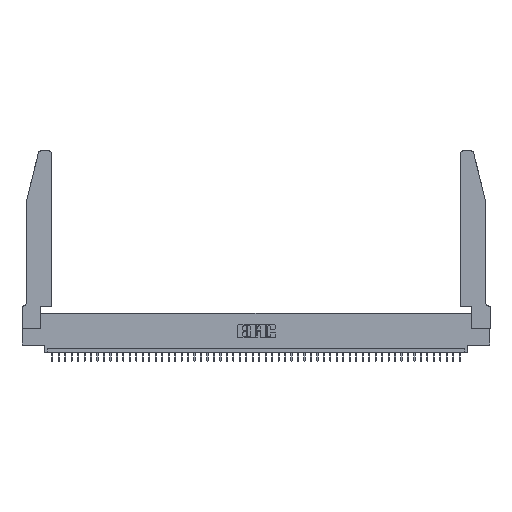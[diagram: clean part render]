
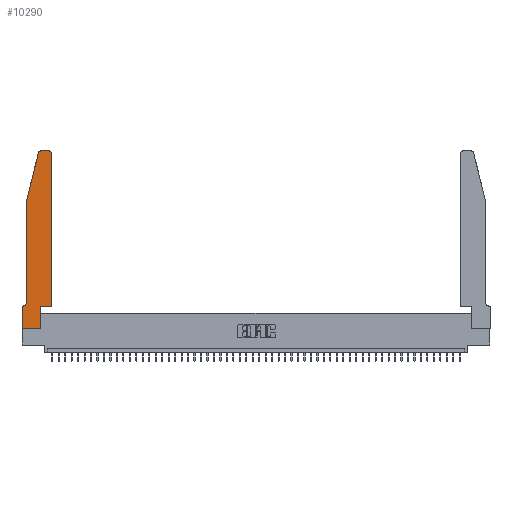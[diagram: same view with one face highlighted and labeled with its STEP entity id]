
A CAD part, top view. The second image highlights one B-rep face of the part: STEP entity #10290.
In plain terms, the highlighted planar face has unit normal (0, 0, 1).
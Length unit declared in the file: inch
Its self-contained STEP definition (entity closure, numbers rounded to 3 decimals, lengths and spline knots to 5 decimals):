
#46 = VECTOR ( 'NONE', #41802, 39.37008 ) ;
#1073 = VECTOR ( 'NONE', #48157, 39.37008 ) ;
#1938 = CARTESIAN_POINT ( 'NONE',  ( 0.2865, 0.35, 0.37 ) ) ;
#2012 = CARTESIAN_POINT ( 'NONE',  ( 0., 0.35, 0.37 ) ) ;
#2520 = VERTEX_POINT ( 'NONE', #20907 ) ;
#2843 = VERTEX_POINT ( 'NONE', #37907 ) ;
#3759 = EDGE_CURVE ( 'NONE', #44016, #2843, #11005, .T. ) ;
#5109 = VECTOR ( 'NONE', #26558, 39.37008 ) ;
#6058 = FACE_OUTER_BOUND ( 'NONE', #34387, .T. ) ;
#6128 = EDGE_CURVE ( 'NONE', #6857, #20717, #10007, .T. ) ;
#6669 = VERTEX_POINT ( 'NONE', #6891 ) ;
#6696 = AXIS2_PLACEMENT_3D ( 'NONE', #35033, #38353, #7597 ) ;
#6857 = VERTEX_POINT ( 'NONE', #25668 ) ;
#6891 = CARTESIAN_POINT ( 'NONE',  ( 0.25487, 2.72718, 0.37 ) ) ;
#6933 = CARTESIAN_POINT ( 'NONE',  ( 0.0755, 2., 0.37 ) ) ;
#7264 = DIRECTION ( 'NONE',  ( 0., 1., 0. ) ) ;
#7509 = ORIENTED_EDGE ( 'NONE', *, *, #19152, .T. ) ;
#7597 = DIRECTION ( 'NONE',  ( 1., 0., 0. ) ) ;
#8338 = ORIENTED_EDGE ( 'NONE', *, *, #40471, .T. ) ;
#8549 = VECTOR ( 'NONE', #49089, 39.37008 ) ;
#8904 = AXIS2_PLACEMENT_3D ( 'NONE', #31086, #23251, #12030 ) ;
#9555 = CARTESIAN_POINT ( 'NONE',  ( 0.4505, 0.35, 0.37 ) ) ;
#10007 = LINE ( 'NONE', #14087, #23589 ) ;
#10290 = ADVANCED_FACE ( 'NONE', ( #6058 ), #36822, .T. ) ;
#11005 = LINE ( 'NONE', #6933, #32248 ) ;
#12030 = DIRECTION ( 'NONE',  ( 1., 0., 0. ) ) ;
#12547 = CARTESIAN_POINT ( 'NONE',  ( 0.2865, 0., 0.37 ) ) ;
#13340 = EDGE_CURVE ( 'NONE', #2520, #31017, #27591, .T. ) ;
#14087 = CARTESIAN_POINT ( 'NONE',  ( 0., 0., 0.37 ) ) ;
#16079 = DIRECTION ( 'NONE',  ( -1., 0., 0. ) ) ;
#16494 = ORIENTED_EDGE ( 'NONE', *, *, #3759, .T. ) ;
#16759 = DIRECTION ( 'NONE',  ( 1., 0., 0. ) ) ;
#17531 = CIRCLE ( 'NONE', #49150, 0.07 ) ;
#17590 = CARTESIAN_POINT ( 'NONE',  ( 0.4505, 0.35, 0.37 ) ) ;
#18054 = VECTOR ( 'NONE', #33067, 39.37008 ) ;
#18724 = CARTESIAN_POINT ( 'NONE',  ( 0.0055, 0.42, 0.37 ) ) ;
#19033 = ORIENTED_EDGE ( 'NONE', *, *, #35173, .T. ) ;
#19152 = EDGE_CURVE ( 'NONE', #48917, #32915, #34416, .T. ) ;
#19551 = ORIENTED_EDGE ( 'NONE', *, *, #39757, .T. ) ;
#19602 = VECTOR ( 'NONE', #16079, 39.37008 ) ;
#19843 = CARTESIAN_POINT ( 'NONE',  ( 0.0055, 0.35, 0.37 ) ) ;
#20717 = VERTEX_POINT ( 'NONE', #12547 ) ;
#20907 = CARTESIAN_POINT ( 'NONE',  ( 0.4505, 2.72, 0.37 ) ) ;
#23020 = LINE ( 'NONE', #34917, #46 ) ;
#23251 = DIRECTION ( 'NONE',  ( 0., 0., 1. ) ) ;
#23589 = VECTOR ( 'NONE', #49363, 39.37008 ) ;
#24156 = VERTEX_POINT ( 'NONE', #39076 ) ;
#25668 = CARTESIAN_POINT ( 'NONE',  ( 0., 0., 0.37 ) ) ;
#26558 = DIRECTION ( 'NONE',  ( -1., 0., 0. ) ) ;
#27591 = CIRCLE ( 'NONE', #8904, 0.03 ) ;
#28416 = EDGE_CURVE ( 'NONE', #6669, #44016, #32864, .T. ) ;
#28615 = CIRCLE ( 'NONE', #6696, 0.03 ) ;
#31017 = VERTEX_POINT ( 'NONE', #31880 ) ;
#31086 = CARTESIAN_POINT ( 'NONE',  ( 0.4205, 2.72, 0.37 ) ) ;
#31209 = ORIENTED_EDGE ( 'NONE', *, *, #13340, .T. ) ;
#31309 = ORIENTED_EDGE ( 'NONE', *, *, #28416, .T. ) ;
#31570 = CARTESIAN_POINT ( 'NONE',  ( 0.2605, 2.75, 0.37 ) ) ;
#31880 = CARTESIAN_POINT ( 'NONE',  ( 0.4205, 2.75, 0.37 ) ) ;
#32248 = VECTOR ( 'NONE', #49350, 39.37008 ) ;
#32677 = LINE ( 'NONE', #44604, #1073 ) ;
#32864 = LINE ( 'NONE', #36936, #8549 ) ;
#32915 = VERTEX_POINT ( 'NONE', #45229 ) ;
#33067 = DIRECTION ( 'NONE',  ( 1., 0., 0. ) ) ;
#34271 = CARTESIAN_POINT ( 'NONE',  ( 0.0755, 2., 0.37 ) ) ;
#34387 = EDGE_LOOP ( 'NONE', ( #38650, #19551, #31309, #16494, #44761, #7509, #19033, #42016, #8338, #45963, #37412, #31209 ) ) ;
#34416 = LINE ( 'NONE', #37974, #5109 ) ;
#34711 = LINE ( 'NONE', #49193, #45926 ) ;
#34917 = CARTESIAN_POINT ( 'NONE',  ( 0., 0., 0.37 ) ) ;
#35033 = CARTESIAN_POINT ( 'NONE',  ( 0.284, 2.72, 0.37 ) ) ;
#35173 = EDGE_CURVE ( 'NONE', #32915, #6857, #23020, .T. ) ;
#36822 = PLANE ( 'NONE',  #45230 ) ;
#36936 = CARTESIAN_POINT ( 'NONE',  ( 0.0755, 2., 0.37 ) ) ;
#37412 = ORIENTED_EDGE ( 'NONE', *, *, #45653, .T. ) ;
#37907 = CARTESIAN_POINT ( 'NONE',  ( 0.0755, 0.42, 0.37 ) ) ;
#37974 = CARTESIAN_POINT ( 'NONE',  ( 0.0755, 0.35, 0.37 ) ) ;
#38353 = DIRECTION ( 'NONE',  ( 0., 0., 1. ) ) ;
#38650 = ORIENTED_EDGE ( 'NONE', *, *, #48600, .T. ) ;
#38900 = EDGE_CURVE ( 'NONE', #40502, #40506, #40430, .T. ) ;
#39076 = CARTESIAN_POINT ( 'NONE',  ( 0.284, 2.75, 0.37 ) ) ;
#39757 = EDGE_CURVE ( 'NONE', #24156, #6669, #28615, .T. ) ;
#40430 = LINE ( 'NONE', #17590, #18054 ) ;
#40471 = EDGE_CURVE ( 'NONE', #20717, #40502, #32677, .T. ) ;
#40502 = VERTEX_POINT ( 'NONE', #1938 ) ;
#40506 = VERTEX_POINT ( 'NONE', #9555 ) ;
#41802 = DIRECTION ( 'NONE',  ( 0., -1., 0. ) ) ;
#42016 = ORIENTED_EDGE ( 'NONE', *, *, #6128, .T. ) ;
#43129 = EDGE_CURVE ( 'NONE', #2843, #48917, #17531, .T. ) ;
#43909 = DIRECTION ( 'NONE',  ( 0., 0., 1. ) ) ;
#44016 = VERTEX_POINT ( 'NONE', #34271 ) ;
#44604 = CARTESIAN_POINT ( 'NONE',  ( 0.2865, 0.35, 0.37 ) ) ;
#44761 = ORIENTED_EDGE ( 'NONE', *, *, #43129, .T. ) ;
#45229 = CARTESIAN_POINT ( 'NONE',  ( 0., 0.35, 0.37 ) ) ;
#45230 = AXIS2_PLACEMENT_3D ( 'NONE', #2012, #43909, #16759 ) ;
#45653 = EDGE_CURVE ( 'NONE', #40506, #2520, #34711, .T. ) ;
#45926 = VECTOR ( 'NONE', #7264, 39.37008 ) ;
#45963 = ORIENTED_EDGE ( 'NONE', *, *, #38900, .T. ) ;
#46108 = DIRECTION ( 'NONE',  ( -1., 0., 0. ) ) ;
#46358 = DIRECTION ( 'NONE',  ( 0., 0., -1. ) ) ;
#46554 = LINE ( 'NONE', #31570, #19602 ) ;
#48157 = DIRECTION ( 'NONE',  ( 0., 1., 0. ) ) ;
#48600 = EDGE_CURVE ( 'NONE', #31017, #24156, #46554, .T. ) ;
#48917 = VERTEX_POINT ( 'NONE', #19843 ) ;
#49089 = DIRECTION ( 'NONE',  ( -0.239, -0.971, 0. ) ) ;
#49150 = AXIS2_PLACEMENT_3D ( 'NONE', #18724, #46358, #46108 ) ;
#49193 = CARTESIAN_POINT ( 'NONE',  ( 0.4505, 0.35, 0.37 ) ) ;
#49350 = DIRECTION ( 'NONE',  ( 0., -1., 0. ) ) ;
#49363 = DIRECTION ( 'NONE',  ( 1., 0., 0. ) ) ;
